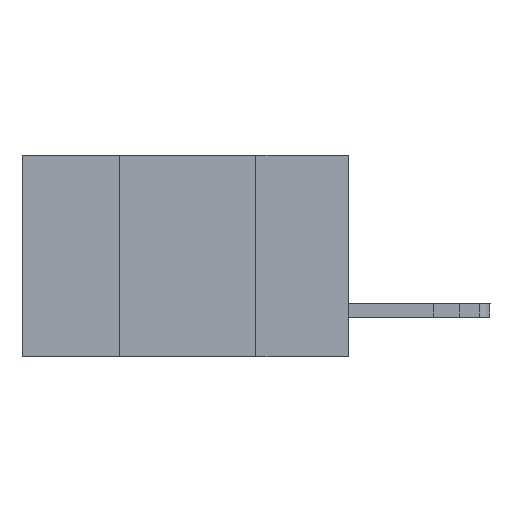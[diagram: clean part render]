
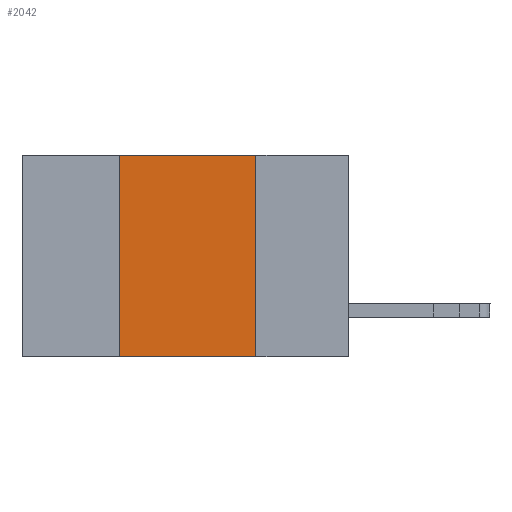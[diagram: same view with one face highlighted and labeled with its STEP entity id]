
A CAD part, left-side view. The second image highlights one B-rep face of the part: STEP entity #2042.
In plain terms, the highlighted planar face has unit normal (-1, 0, 0).
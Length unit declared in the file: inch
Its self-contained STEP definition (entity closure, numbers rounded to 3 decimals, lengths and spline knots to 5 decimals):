
#65 = VECTOR ( 'NONE', #5144, 39.37008 ) ;
#167 = DIRECTION ( 'NONE',  ( 0., -1., 0. ) ) ;
#209 = LINE ( 'NONE', #7445, #7296 ) ;
#364 = VERTEX_POINT ( 'NONE', #10233 ) ;
#627 = LINE ( 'NONE', #4275, #65 ) ;
#726 = EDGE_CURVE ( 'NONE', #364, #3253, #3884, .T. ) ;
#799 = AXIS2_PLACEMENT_3D ( 'NONE', #4878, #4860, #4761 ) ;
#938 = CARTESIAN_POINT ( 'NONE',  ( 0., 0.17, -0.37 ) ) ;
#989 = CARTESIAN_POINT ( 'NONE',  ( 0., 0.6, -0.37 ) ) ;
#1294 = CARTESIAN_POINT ( 'NONE',  ( 0., 0.6, 0. ) ) ;
#2042 = ADVANCED_FACE ( 'NONE', ( #9369 ), #5015, .F. ) ;
#2734 = EDGE_LOOP ( 'NONE', ( #8854, #11274, #4325, #7234 ) ) ;
#3219 = CARTESIAN_POINT ( 'NONE',  ( 0., 0.17, 0. ) ) ;
#3253 = VERTEX_POINT ( 'NONE', #938 ) ;
#3606 = EDGE_CURVE ( 'NONE', #3995, #3253, #209, .T. ) ;
#3884 = LINE ( 'NONE', #989, #10406 ) ;
#3995 = VERTEX_POINT ( 'NONE', #3219 ) ;
#4076 = DIRECTION ( 'NONE',  ( 0., -1., 0. ) ) ;
#4275 = CARTESIAN_POINT ( 'NONE',  ( 0., 0.42, -0.37 ) ) ;
#4325 = ORIENTED_EDGE ( 'NONE', *, *, #10877, .F. ) ;
#4761 = DIRECTION ( 'NONE',  ( 0., 0., -1. ) ) ;
#4837 = VECTOR ( 'NONE', #4076, 39.37008 ) ;
#4860 = DIRECTION ( 'NONE',  ( 1., 0., 0. ) ) ;
#4878 = CARTESIAN_POINT ( 'NONE',  ( 0., 0.6, 0. ) ) ;
#5015 = PLANE ( 'NONE',  #799 ) ;
#5144 = DIRECTION ( 'NONE',  ( 0., 0., 1. ) ) ;
#5784 = VERTEX_POINT ( 'NONE', #6369 ) ;
#6369 = CARTESIAN_POINT ( 'NONE',  ( 0., 0.42, 0. ) ) ;
#7234 = ORIENTED_EDGE ( 'NONE', *, *, #726, .T. ) ;
#7296 = VECTOR ( 'NONE', #7498, 39.37008 ) ;
#7445 = CARTESIAN_POINT ( 'NONE',  ( 0., 0.17, -0.37 ) ) ;
#7498 = DIRECTION ( 'NONE',  ( 0., 0., -1. ) ) ;
#8854 = ORIENTED_EDGE ( 'NONE', *, *, #3606, .F. ) ;
#9223 = EDGE_CURVE ( 'NONE', #5784, #3995, #9367, .T. ) ;
#9367 = LINE ( 'NONE', #1294, #4837 ) ;
#9369 = FACE_OUTER_BOUND ( 'NONE', #2734, .T. ) ;
#10233 = CARTESIAN_POINT ( 'NONE',  ( 0., 0.42, -0.37 ) ) ;
#10406 = VECTOR ( 'NONE', #167, 39.37008 ) ;
#10877 = EDGE_CURVE ( 'NONE', #364, #5784, #627, .T. ) ;
#11274 = ORIENTED_EDGE ( 'NONE', *, *, #9223, .F. ) ;
